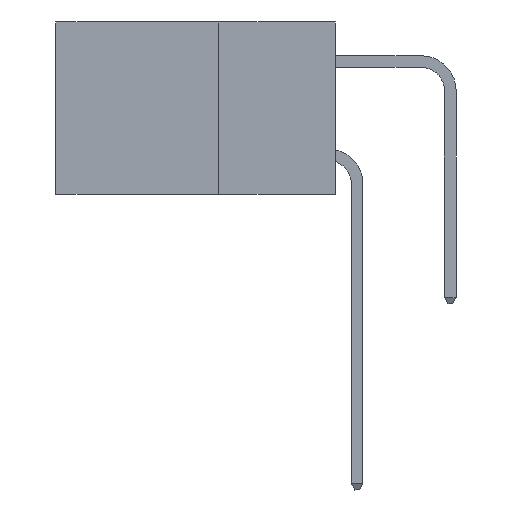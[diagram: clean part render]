
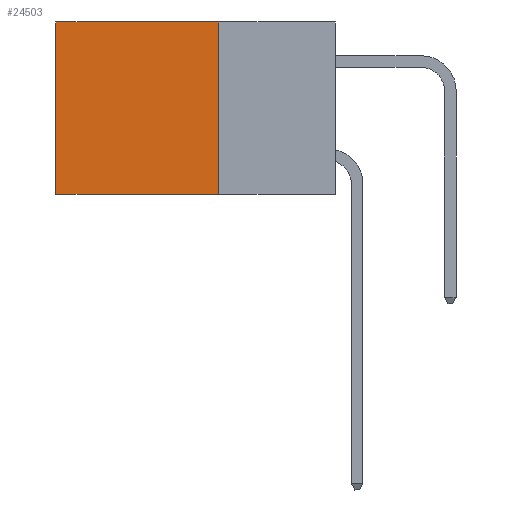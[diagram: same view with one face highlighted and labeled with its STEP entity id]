
A CAD part, left-side view. The second image highlights one B-rep face of the part: STEP entity #24503.
In plain terms, the highlighted planar face has unit normal (-1, 0, 0).
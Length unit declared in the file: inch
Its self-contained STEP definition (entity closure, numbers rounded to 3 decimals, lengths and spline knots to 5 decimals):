
#708 = CARTESIAN_POINT ( 'NONE',  ( 0.2875, 0.6, 0. ) ) ;
#2555 = CARTESIAN_POINT ( 'NONE',  ( 0.2875, 0.25, 0. ) ) ;
#3108 = CARTESIAN_POINT ( 'NONE',  ( 0.2875, 0.25, 0. ) ) ;
#3283 = ORIENTED_EDGE ( 'NONE', *, *, #4400, .F. ) ;
#4400 = EDGE_CURVE ( 'NONE', #6400, #13408, #23163, .T. ) ;
#4652 = CARTESIAN_POINT ( 'NONE',  ( 0.2875, 0.6, -0.37 ) ) ;
#5736 = ORIENTED_EDGE ( 'NONE', *, *, #13931, .T. ) ;
#5798 = DIRECTION ( 'NONE',  ( 0., 0., -1. ) ) ;
#5834 = AXIS2_PLACEMENT_3D ( 'NONE', #3108, #15358, #36793 ) ;
#6205 = DIRECTION ( 'NONE',  ( 0., 1., 0. ) ) ;
#6400 = VERTEX_POINT ( 'NONE', #32672 ) ;
#7230 = ORIENTED_EDGE ( 'NONE', *, *, #13512, .T. ) ;
#7731 = VERTEX_POINT ( 'NONE', #708 ) ;
#10611 = LINE ( 'NONE', #2555, #30359 ) ;
#11829 = VERTEX_POINT ( 'NONE', #31015 ) ;
#13408 = VERTEX_POINT ( 'NONE', #4652 ) ;
#13512 = EDGE_CURVE ( 'NONE', #7731, #13408, #26127, .T. ) ;
#13931 = EDGE_CURVE ( 'NONE', #11829, #7731, #39546, .T. ) ;
#15358 = DIRECTION ( 'NONE',  ( 1., 0., 0. ) ) ;
#18034 = CARTESIAN_POINT ( 'NONE',  ( 0.2875, 0.25, -0.37 ) ) ;
#18411 = FACE_OUTER_BOUND ( 'NONE', #24601, .T. ) ;
#18691 = CARTESIAN_POINT ( 'NONE',  ( 0.2875, 0.6, 0. ) ) ;
#23163 = LINE ( 'NONE', #18034, #38569 ) ;
#24100 = DIRECTION ( 'NONE',  ( 0., 0., -1. ) ) ;
#24503 = ADVANCED_FACE ( 'NONE', ( #18411 ), #30872, .F. ) ;
#24601 = EDGE_LOOP ( 'NONE', ( #7230, #3283, #31165, #5736 ) ) ;
#26127 = LINE ( 'NONE', #18691, #34801 ) ;
#29614 = DIRECTION ( 'NONE',  ( 0., 1., 0. ) ) ;
#30359 = VECTOR ( 'NONE', #24100, 39.37008 ) ;
#30872 = PLANE ( 'NONE',  #5834 ) ;
#31015 = CARTESIAN_POINT ( 'NONE',  ( 0.2875, 0.25, 0. ) ) ;
#31165 = ORIENTED_EDGE ( 'NONE', *, *, #39335, .F. ) ;
#31403 = VECTOR ( 'NONE', #29614, 39.37008 ) ;
#32672 = CARTESIAN_POINT ( 'NONE',  ( 0.2875, 0.25, -0.37 ) ) ;
#34801 = VECTOR ( 'NONE', #5798, 39.37008 ) ;
#35927 = CARTESIAN_POINT ( 'NONE',  ( 0.2875, 0.25, 0. ) ) ;
#36793 = DIRECTION ( 'NONE',  ( 0., 0., -1. ) ) ;
#38569 = VECTOR ( 'NONE', #6205, 39.37008 ) ;
#39335 = EDGE_CURVE ( 'NONE', #11829, #6400, #10611, .T. ) ;
#39546 = LINE ( 'NONE', #35927, #31403 ) ;
